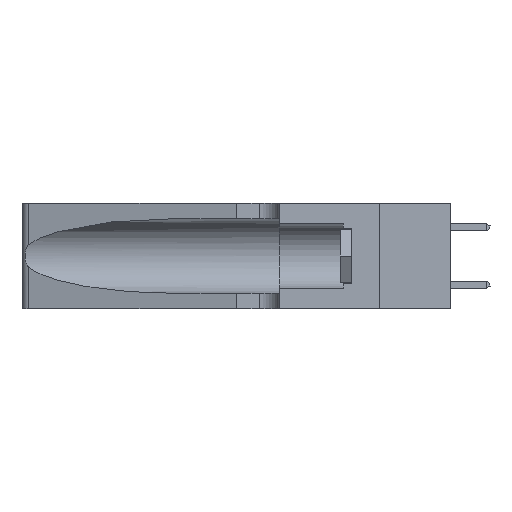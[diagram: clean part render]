
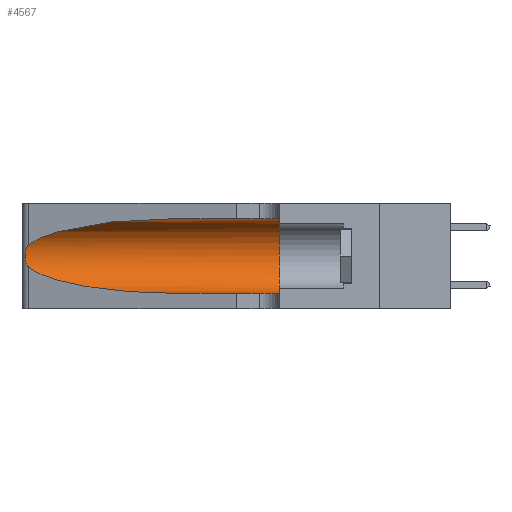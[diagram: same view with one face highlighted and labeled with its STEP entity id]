
A CAD part, left-side view. The second image highlights one B-rep face of the part: STEP entity #4567.
In plain terms, the highlighted cylindrical face has radius 3.308 mm (diameter 6.617 mm), a partial arc.
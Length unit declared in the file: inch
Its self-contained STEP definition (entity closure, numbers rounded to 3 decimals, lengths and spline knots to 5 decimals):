
#285 = DIRECTION ( 'NONE',  ( 0., 1., 0. ) ) ;
#842 =( BOUNDED_CURVE ( )  B_SPLINE_CURVE ( 3, ( #15232, #4034, #7350, #18385 ),
 .UNSPECIFIED., .F., .T. ) 
 B_SPLINE_CURVE_WITH_KNOTS ( ( 4, 4 ),
 ( 1.5708, 2.84003 ),
 .UNSPECIFIED. ) 
 CURVE ( )  GEOMETRIC_REPRESENTATION_ITEM ( )  RATIONAL_B_SPLINE_CURVE ( ( 1., 0.87, 0.87, 1. ) ) 
 REPRESENTATION_ITEM ( '' )  );
#936 = VECTOR ( 'NONE', #1376, 39.37008 ) ;
#966 = CARTESIAN_POINT ( 'NONE',  ( 0.25487, 1.22718, 0.22369 ) ) ;
#968 = CARTESIAN_POINT ( 'NONE',  ( 0.1305, 0.35, 0.31525 ) ) ;
#1029 = CARTESIAN_POINT ( 'NONE',  ( 0.18966, 0.96281, 0.05475 ) ) ;
#1376 = DIRECTION ( 'NONE',  ( 0., -1., 0. ) ) ;
#1881 = CARTESIAN_POINT ( 'NONE',  ( 0.25487, 1.22718, 0.14631 ) ) ;
#1943 =( BOUNDED_CURVE ( )  B_SPLINE_CURVE ( 3, ( #9211, #6041, #1029, #12474 ),
 .UNSPECIFIED., .F., .T. ) 
 B_SPLINE_CURVE_WITH_KNOTS ( ( 4, 4 ),
 ( 3.44316, 4.71239 ),
 .UNSPECIFIED. ) 
 CURVE ( )  GEOMETRIC_REPRESENTATION_ITEM ( )  RATIONAL_B_SPLINE_CURVE ( ( 1., 0.87, 0.87, 1. ) ) 
 REPRESENTATION_ITEM ( '' )  );
#2509 = B_SPLINE_CURVE_WITH_KNOTS ( 'NONE', 3,
 ( #966, #9233, #5986, #12425, #2700, #14012, #4400, #15586, #6064, #17182, #7703, #18723, #9303, #20283 ),
 .UNSPECIFIED., .F., .F.,
 ( 4, 2, 2, 2, 2, 2, 4 ),
 ( 0., 0.00027, 0.00053, 0.00107, 0.0016, 0.00187, 0.00214 ),
 .UNSPECIFIED. ) ;
#2639 = CIRCLE ( 'NONE', #6396, 0.13025 ) ;
#2700 = CARTESIAN_POINT ( 'NONE',  ( 0.25854, 1.2359, 0.20912 ) ) ;
#3107 = VERTEX_POINT ( 'NONE', #968 ) ;
#3988 = CARTESIAN_POINT ( 'NONE',  ( 0.1305, 0.35, 0.05475 ) ) ;
#4034 = CARTESIAN_POINT ( 'NONE',  ( 0.18966, 0.96281, 0.31525 ) ) ;
#4400 = CARTESIAN_POINT ( 'NONE',  ( 0.26075, 1.23896, 0.19203 ) ) ;
#4567 = ADVANCED_FACE ( 'NONE', ( #10423 ), #14129, .F. ) ;
#4923 = CARTESIAN_POINT ( 'NONE',  ( 0.1305, 1.61858, 0.05475 ) ) ;
#5317 = VECTOR ( 'NONE', #16095, 39.37008 ) ;
#5545 = ORIENTED_EDGE ( 'NONE', *, *, #18438, .T. ) ;
#5986 = CARTESIAN_POINT ( 'NONE',  ( 0.25639, 1.23184, 0.21858 ) ) ;
#6041 = CARTESIAN_POINT ( 'NONE',  ( 0.2373, 1.15595, 0.08982 ) ) ;
#6064 = CARTESIAN_POINT ( 'NONE',  ( 0.26017, 1.23833, 0.17102 ) ) ;
#6359 = EDGE_CURVE ( 'NONE', #15308, #20051, #2509, .T. ) ;
#6396 = AXIS2_PLACEMENT_3D ( 'NONE', #10182, #285, #11808 ) ;
#6744 = CARTESIAN_POINT ( 'NONE',  ( 0.1305, 0.72297, 0.05475 ) ) ;
#7114 = VERTEX_POINT ( 'NONE', #8243 ) ;
#7350 = CARTESIAN_POINT ( 'NONE',  ( 0.2373, 1.15595, 0.28018 ) ) ;
#7703 = CARTESIAN_POINT ( 'NONE',  ( 0.25789, 1.23486, 0.15765 ) ) ;
#8243 = CARTESIAN_POINT ( 'NONE',  ( 0.1305, 0.72297, 0.31525 ) ) ;
#8374 = ORIENTED_EDGE ( 'NONE', *, *, #9393, .T. ) ;
#9211 = CARTESIAN_POINT ( 'NONE',  ( 0.25487, 1.22718, 0.14631 ) ) ;
#9233 = CARTESIAN_POINT ( 'NONE',  ( 0.25555, 1.22994, 0.2215 ) ) ;
#9303 = CARTESIAN_POINT ( 'NONE',  ( 0.25555, 1.22993, 0.14849 ) ) ;
#9393 = EDGE_CURVE ( 'NONE', #9475, #13966, #13821, .T. ) ;
#9475 = VERTEX_POINT ( 'NONE', #6744 ) ;
#10182 = CARTESIAN_POINT ( 'NONE',  ( 0.1305, 0.35, 0.185 ) ) ;
#10423 = FACE_OUTER_BOUND ( 'NONE', #10776, .T. ) ;
#10776 = EDGE_LOOP ( 'NONE', ( #5545, #12331, #18012, #8374, #13575, #18244 ) ) ;
#11376 = DIRECTION ( 'NONE',  ( 0., -1., 0. ) ) ;
#11808 = DIRECTION ( 'NONE',  ( 0., 0., 1. ) ) ;
#11976 = AXIS2_PLACEMENT_3D ( 'NONE', #20735, #11376, #19179 ) ;
#12331 = ORIENTED_EDGE ( 'NONE', *, *, #6359, .T. ) ;
#12425 = CARTESIAN_POINT ( 'NONE',  ( 0.25787, 1.23484, 0.2124 ) ) ;
#12474 = CARTESIAN_POINT ( 'NONE',  ( 0.1305, 0.72297, 0.05475 ) ) ;
#12938 = EDGE_CURVE ( 'NONE', #20051, #9475, #1943, .T. ) ;
#13575 = ORIENTED_EDGE ( 'NONE', *, *, #16842, .F. ) ;
#13627 = CARTESIAN_POINT ( 'NONE',  ( 0.25487, 1.22718, 0.22369 ) ) ;
#13821 = LINE ( 'NONE', #4923, #5317 ) ;
#13966 = VERTEX_POINT ( 'NONE', #3988 ) ;
#14012 = CARTESIAN_POINT ( 'NONE',  ( 0.26018, 1.23835, 0.19895 ) ) ;
#14129 = CYLINDRICAL_SURFACE ( 'NONE', #11976, 0.13025 ) ;
#15232 = CARTESIAN_POINT ( 'NONE',  ( 0.1305, 0.72297, 0.31525 ) ) ;
#15308 = VERTEX_POINT ( 'NONE', #13627 ) ;
#15586 = CARTESIAN_POINT ( 'NONE',  ( 0.26075, 1.23896, 0.178 ) ) ;
#16095 = DIRECTION ( 'NONE',  ( 0., -1., 0. ) ) ;
#16842 = EDGE_CURVE ( 'NONE', #3107, #13966, #2639, .T. ) ;
#17182 = CARTESIAN_POINT ( 'NONE',  ( 0.25856, 1.23593, 0.16098 ) ) ;
#18012 = ORIENTED_EDGE ( 'NONE', *, *, #12938, .T. ) ;
#18137 = LINE ( 'NONE', #20571, #936 ) ;
#18244 = ORIENTED_EDGE ( 'NONE', *, *, #19334, .F. ) ;
#18385 = CARTESIAN_POINT ( 'NONE',  ( 0.25487, 1.22718, 0.22369 ) ) ;
#18438 = EDGE_CURVE ( 'NONE', #7114, #15308, #842, .T. ) ;
#18723 = CARTESIAN_POINT ( 'NONE',  ( 0.25639, 1.23186, 0.15144 ) ) ;
#19179 = DIRECTION ( 'NONE',  ( 0., 0., -1. ) ) ;
#19334 = EDGE_CURVE ( 'NONE', #7114, #3107, #18137, .T. ) ;
#20051 = VERTEX_POINT ( 'NONE', #1881 ) ;
#20283 = CARTESIAN_POINT ( 'NONE',  ( 0.25487, 1.22718, 0.14631 ) ) ;
#20571 = CARTESIAN_POINT ( 'NONE',  ( 0.1305, 1.61858, 0.31525 ) ) ;
#20735 = CARTESIAN_POINT ( 'NONE',  ( 0.1305, 1.61858, 0.185 ) ) ;
